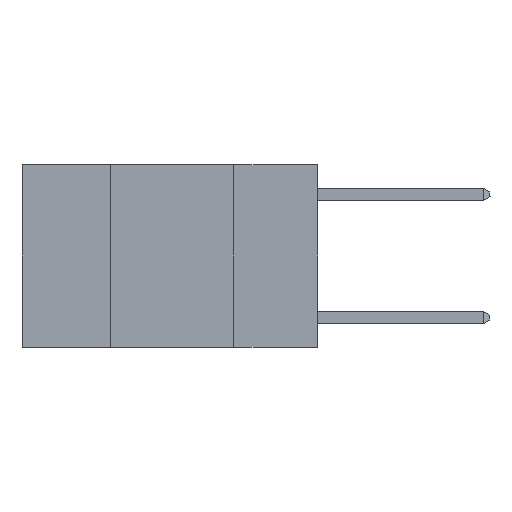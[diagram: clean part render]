
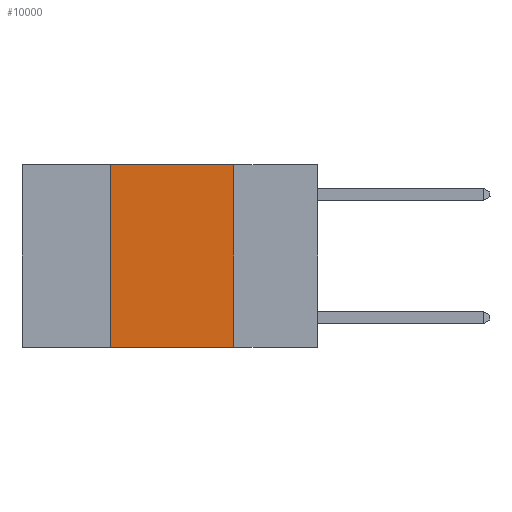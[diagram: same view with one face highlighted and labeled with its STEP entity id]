
A CAD part, left-side view. The second image highlights one B-rep face of the part: STEP entity #10000.
In plain terms, the highlighted planar face has unit normal (-1, 0, 0).
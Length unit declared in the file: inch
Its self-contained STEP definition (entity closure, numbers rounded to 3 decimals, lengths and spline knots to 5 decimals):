
#122 = VERTEX_POINT ( 'NONE', #10174 ) ;
#1447 = CARTESIAN_POINT ( 'NONE',  ( 0., 0.17, 0. ) ) ;
#1695 = VECTOR ( 'NONE', #3024, 39.37008 ) ;
#1837 = LINE ( 'NONE', #3669, #8579 ) ;
#2801 = PLANE ( 'NONE',  #6471 ) ;
#3024 = DIRECTION ( 'NONE',  ( 0., -1., 0. ) ) ;
#3109 = LINE ( 'NONE', #1447, #7647 ) ;
#3388 = EDGE_LOOP ( 'NONE', ( #3517, #9586, #10198, #7090 ) ) ;
#3472 = EDGE_CURVE ( 'NONE', #4352, #122, #4227, .T. ) ;
#3517 = ORIENTED_EDGE ( 'NONE', *, *, #5264, .F. ) ;
#3633 = DIRECTION ( 'NONE',  ( 0., 0., 1. ) ) ;
#3669 = CARTESIAN_POINT ( 'NONE',  ( 0., 0.42, 0. ) ) ;
#3942 = DIRECTION ( 'NONE',  ( 0., -1., 0. ) ) ;
#4190 = LINE ( 'NONE', #7294, #8428 ) ;
#4227 = LINE ( 'NONE', #5566, #1695 ) ;
#4352 = VERTEX_POINT ( 'NONE', #7049 ) ;
#4557 = DIRECTION ( 'NONE',  ( 0., 0., -1. ) ) ;
#4685 = VERTEX_POINT ( 'NONE', #4697 ) ;
#4697 = CARTESIAN_POINT ( 'NONE',  ( 0., 0.42, 0. ) ) ;
#4898 = CARTESIAN_POINT ( 'NONE',  ( 0., 0.17, 0. ) ) ;
#5264 = EDGE_CURVE ( 'NONE', #9304, #122, #3109, .T. ) ;
#5531 = EDGE_CURVE ( 'NONE', #4352, #4685, #1837, .T. ) ;
#5566 = CARTESIAN_POINT ( 'NONE',  ( 0., 0.6, -0.37 ) ) ;
#5785 = EDGE_CURVE ( 'NONE', #4685, #9304, #4190, .T. ) ;
#6471 = AXIS2_PLACEMENT_3D ( 'NONE', #8836, #9630, #4557 ) ;
#7049 = CARTESIAN_POINT ( 'NONE',  ( 0., 0.42, -0.37 ) ) ;
#7090 = ORIENTED_EDGE ( 'NONE', *, *, #3472, .T. ) ;
#7294 = CARTESIAN_POINT ( 'NONE',  ( 0., 0.6, 0. ) ) ;
#7647 = VECTOR ( 'NONE', #10144, 39.37008 ) ;
#8428 = VECTOR ( 'NONE', #3942, 39.37008 ) ;
#8579 = VECTOR ( 'NONE', #3633, 39.37008 ) ;
#8836 = CARTESIAN_POINT ( 'NONE',  ( 0., 0.6, 0. ) ) ;
#9304 = VERTEX_POINT ( 'NONE', #4898 ) ;
#9586 = ORIENTED_EDGE ( 'NONE', *, *, #5785, .F. ) ;
#9630 = DIRECTION ( 'NONE',  ( 1., 0., 0. ) ) ;
#9800 = FACE_OUTER_BOUND ( 'NONE', #3388, .T. ) ;
#10000 = ADVANCED_FACE ( 'NONE', ( #9800 ), #2801, .F. ) ;
#10144 = DIRECTION ( 'NONE',  ( 0., 0., -1. ) ) ;
#10174 = CARTESIAN_POINT ( 'NONE',  ( 0., 0.17, -0.37 ) ) ;
#10198 = ORIENTED_EDGE ( 'NONE', *, *, #5531, .F. ) ;
